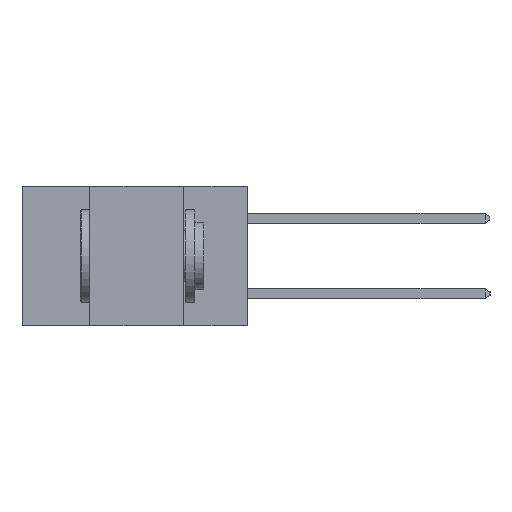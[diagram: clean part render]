
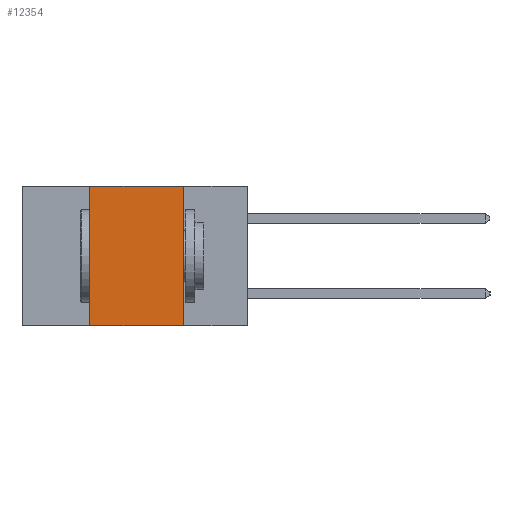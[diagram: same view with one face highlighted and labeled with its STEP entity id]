
A CAD part, left-side view. The second image highlights one B-rep face of the part: STEP entity #12354.
In plain terms, the highlighted planar face has unit normal (-1, 0, 0).
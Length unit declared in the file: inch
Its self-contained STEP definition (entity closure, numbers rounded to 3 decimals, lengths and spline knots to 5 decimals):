
#1171 = AXIS2_PLACEMENT_3D ( 'NONE', #15064, #4817, #19144 ) ;
#2398 = VECTOR ( 'NONE', #23301, 39.37008 ) ;
#2771 = CARTESIAN_POINT ( 'NONE',  ( 0., 0.6, 0. ) ) ;
#3297 = EDGE_CURVE ( 'NONE', #4251, #10409, #24036, .T. ) ;
#3460 = EDGE_CURVE ( 'NONE', #4251, #14687, #10789, .T. ) ;
#4251 = VERTEX_POINT ( 'NONE', #9879 ) ;
#4817 = DIRECTION ( 'NONE',  ( 1., 0., 0. ) ) ;
#5047 = EDGE_CURVE ( 'NONE', #10290, #14687, #19619, .T. ) ;
#5816 = FACE_OUTER_BOUND ( 'NONE', #21301, .T. ) ;
#6271 = ORIENTED_EDGE ( 'NONE', *, *, #5047, .F. ) ;
#6356 = CARTESIAN_POINT ( 'NONE',  ( 0., 0.17, -0.37 ) ) ;
#6592 = DIRECTION ( 'NONE',  ( 0., 0., -1. ) ) ;
#7792 = ORIENTED_EDGE ( 'NONE', *, *, #9548, .F. ) ;
#8013 = ORIENTED_EDGE ( 'NONE', *, *, #3297, .F. ) ;
#9548 = EDGE_CURVE ( 'NONE', #10409, #10290, #22893, .T. ) ;
#9879 = CARTESIAN_POINT ( 'NONE',  ( 0., 0.42, -0.37 ) ) ;
#10290 = VERTEX_POINT ( 'NONE', #25105 ) ;
#10409 = VERTEX_POINT ( 'NONE', #23462 ) ;
#10789 = LINE ( 'NONE', #13293, #20303 ) ;
#11059 = DIRECTION ( 'NONE',  ( 0., -1., 0. ) ) ;
#12354 = ADVANCED_FACE ( 'NONE', ( #5816 ), #25059, .F. ) ;
#13293 = CARTESIAN_POINT ( 'NONE',  ( 0., 0.6, -0.37 ) ) ;
#13375 = DIRECTION ( 'NONE',  ( 0., -1., 0. ) ) ;
#13581 = CARTESIAN_POINT ( 'NONE',  ( 0., 0.17, -0.37 ) ) ;
#14687 = VERTEX_POINT ( 'NONE', #13581 ) ;
#15064 = CARTESIAN_POINT ( 'NONE',  ( 0., 0.6, 0. ) ) ;
#17559 = VECTOR ( 'NONE', #11059, 39.37008 ) ;
#19144 = DIRECTION ( 'NONE',  ( 0., 0., -1. ) ) ;
#19619 = LINE ( 'NONE', #6356, #24290 ) ;
#20303 = VECTOR ( 'NONE', #13375, 39.37008 ) ;
#21129 = ORIENTED_EDGE ( 'NONE', *, *, #3460, .T. ) ;
#21301 = EDGE_LOOP ( 'NONE', ( #6271, #7792, #8013, #21129 ) ) ;
#22893 = LINE ( 'NONE', #2771, #17559 ) ;
#23301 = DIRECTION ( 'NONE',  ( 0., 0., 1. ) ) ;
#23462 = CARTESIAN_POINT ( 'NONE',  ( 0., 0.42, 0. ) ) ;
#24021 = CARTESIAN_POINT ( 'NONE',  ( 0., 0.42, -0.37 ) ) ;
#24036 = LINE ( 'NONE', #24021, #2398 ) ;
#24290 = VECTOR ( 'NONE', #6592, 39.37008 ) ;
#25059 = PLANE ( 'NONE',  #1171 ) ;
#25105 = CARTESIAN_POINT ( 'NONE',  ( 0., 0.17, 0. ) ) ;
